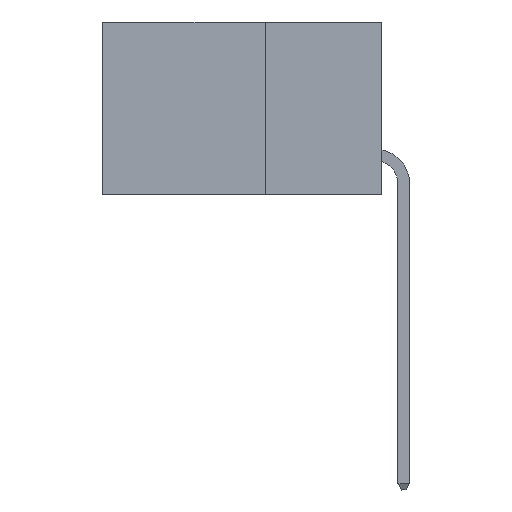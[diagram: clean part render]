
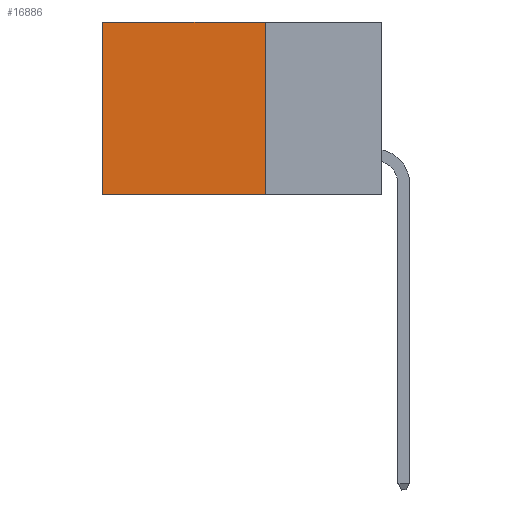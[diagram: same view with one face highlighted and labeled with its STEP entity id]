
A CAD part, left-side view. The second image highlights one B-rep face of the part: STEP entity #16886.
In plain terms, the highlighted planar face has unit normal (-1, 0, 0).
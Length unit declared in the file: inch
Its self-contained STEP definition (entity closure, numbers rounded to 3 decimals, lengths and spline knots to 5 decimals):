
#503 = CARTESIAN_POINT ( 'NONE',  ( 0.2875, 0.6, 0. ) ) ;
#876 = VECTOR ( 'NONE', #29670, 39.37008 ) ;
#1807 = DIRECTION ( 'NONE',  ( 0., 1., 0. ) ) ;
#2171 = LINE ( 'NONE', #24201, #9614 ) ;
#3382 = PLANE ( 'NONE',  #38927 ) ;
#5879 = EDGE_CURVE ( 'NONE', #7340, #36507, #6849, .T. ) ;
#6849 = LINE ( 'NONE', #29942, #876 ) ;
#7340 = VERTEX_POINT ( 'NONE', #31342 ) ;
#7439 = EDGE_LOOP ( 'NONE', ( #14685, #13586, #10029, #35224 ) ) ;
#9196 = EDGE_CURVE ( 'NONE', #36507, #32713, #2171, .T. ) ;
#9434 = LINE ( 'NONE', #503, #26457 ) ;
#9614 = VECTOR ( 'NONE', #1807, 39.37008 ) ;
#10029 = ORIENTED_EDGE ( 'NONE', *, *, #5879, .F. ) ;
#13586 = ORIENTED_EDGE ( 'NONE', *, *, #9196, .F. ) ;
#14685 = ORIENTED_EDGE ( 'NONE', *, *, #27270, .T. ) ;
#16886 = ADVANCED_FACE ( 'NONE', ( #22768 ), #3382, .F. ) ;
#18998 = VECTOR ( 'NONE', #26025, 39.37008 ) ;
#20241 = CARTESIAN_POINT ( 'NONE',  ( 0.2875, 0.6, 0. ) ) ;
#21808 = EDGE_CURVE ( 'NONE', #7340, #24858, #37113, .T. ) ;
#22768 = FACE_OUTER_BOUND ( 'NONE', #7439, .T. ) ;
#24201 = CARTESIAN_POINT ( 'NONE',  ( 0.2875, 0.25, -0.37 ) ) ;
#24312 = DIRECTION ( 'NONE',  ( 0., 0., -1. ) ) ;
#24858 = VERTEX_POINT ( 'NONE', #20241 ) ;
#25800 = CARTESIAN_POINT ( 'NONE',  ( 0.2875, 0.25, 0. ) ) ;
#26025 = DIRECTION ( 'NONE',  ( 0., 1., 0. ) ) ;
#26457 = VECTOR ( 'NONE', #24312, 39.37008 ) ;
#26459 = DIRECTION ( 'NONE',  ( 0., 0., -1. ) ) ;
#27270 = EDGE_CURVE ( 'NONE', #24858, #32713, #9434, .T. ) ;
#29670 = DIRECTION ( 'NONE',  ( 0., 0., -1. ) ) ;
#29942 = CARTESIAN_POINT ( 'NONE',  ( 0.2875, 0.25, 0. ) ) ;
#31342 = CARTESIAN_POINT ( 'NONE',  ( 0.2875, 0.25, 0. ) ) ;
#31488 = CARTESIAN_POINT ( 'NONE',  ( 0.2875, 0.6, -0.37 ) ) ;
#32713 = VERTEX_POINT ( 'NONE', #31488 ) ;
#32963 = CARTESIAN_POINT ( 'NONE',  ( 0.2875, 0.25, 0. ) ) ;
#33397 = DIRECTION ( 'NONE',  ( 1., 0., 0. ) ) ;
#35224 = ORIENTED_EDGE ( 'NONE', *, *, #21808, .T. ) ;
#36507 = VERTEX_POINT ( 'NONE', #40329 ) ;
#37113 = LINE ( 'NONE', #32963, #18998 ) ;
#38927 = AXIS2_PLACEMENT_3D ( 'NONE', #25800, #33397, #26459 ) ;
#40329 = CARTESIAN_POINT ( 'NONE',  ( 0.2875, 0.25, -0.37 ) ) ;
